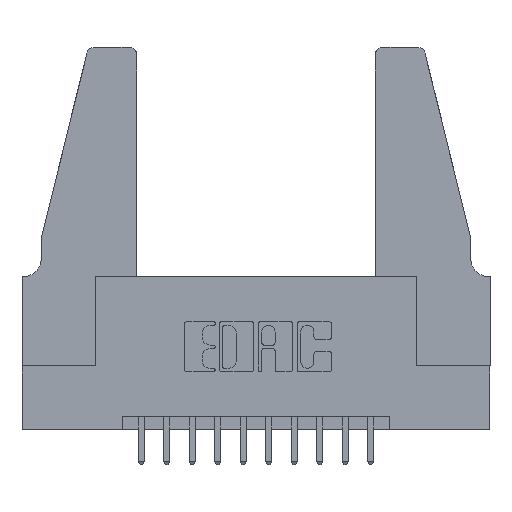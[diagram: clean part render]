
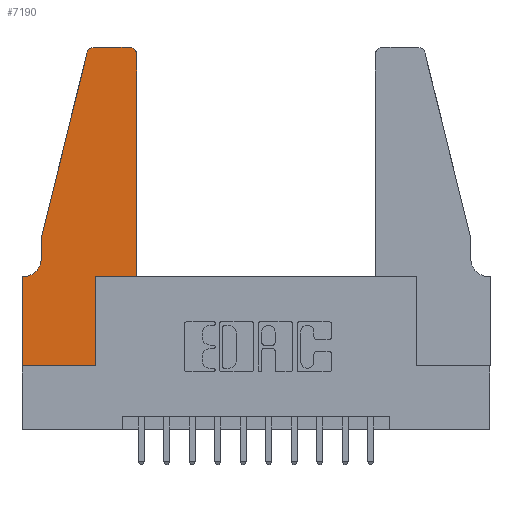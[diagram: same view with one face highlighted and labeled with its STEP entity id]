
A CAD part, top view. The second image highlights one B-rep face of the part: STEP entity #7190.
In plain terms, the highlighted planar face has unit normal (0, 0, 1).
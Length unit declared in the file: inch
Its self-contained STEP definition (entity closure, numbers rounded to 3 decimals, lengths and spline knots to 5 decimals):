
#106 = DIRECTION ( 'NONE',  ( 0., 0., 1. ) ) ;
#136 = CIRCLE ( 'NONE', #2397, 0.03 ) ;
#279 = DIRECTION ( 'NONE',  ( 1., 0., 0. ) ) ;
#528 = CARTESIAN_POINT ( 'NONE',  ( 0.4205, 1.22, 0.37 ) ) ;
#578 = ORIENTED_EDGE ( 'NONE', *, *, #6038, .T. ) ;
#714 = EDGE_CURVE ( 'NONE', #11721, #8937, #3862, .T. ) ;
#1007 = VERTEX_POINT ( 'NONE', #6798 ) ;
#1129 = ORIENTED_EDGE ( 'NONE', *, *, #714, .T. ) ;
#1143 = CARTESIAN_POINT ( 'NONE',  ( 0.2605, 1.25, 0.37 ) ) ;
#1186 = CIRCLE ( 'NONE', #14248, 0.03 ) ;
#1503 = LINE ( 'NONE', #11386, #5485 ) ;
#1522 = DIRECTION ( 'NONE',  ( 0., 0., 1. ) ) ;
#1539 = CARTESIAN_POINT ( 'NONE',  ( 0.0755, 0.42, 0.37 ) ) ;
#1570 = VECTOR ( 'NONE', #9834, 39.37008 ) ;
#1908 = VECTOR ( 'NONE', #6841, 39.37008 ) ;
#2187 = DIRECTION ( 'NONE',  ( 1., 0., 0. ) ) ;
#2288 = CARTESIAN_POINT ( 'NONE',  ( 0.0755, 0.5, 0.37 ) ) ;
#2299 = CARTESIAN_POINT ( 'NONE',  ( 0.25487, 1.22718, 0.37 ) ) ;
#2397 = AXIS2_PLACEMENT_3D ( 'NONE', #528, #12698, #13999 ) ;
#2449 = LINE ( 'NONE', #9709, #11997 ) ;
#2630 = CARTESIAN_POINT ( 'NONE',  ( 0., 0., 0.37 ) ) ;
#2727 = ORIENTED_EDGE ( 'NONE', *, *, #8529, .T. ) ;
#2796 = CARTESIAN_POINT ( 'NONE',  ( 0.284, 1.25, 0.37 ) ) ;
#3583 = VERTEX_POINT ( 'NONE', #2299 ) ;
#3639 = EDGE_CURVE ( 'NONE', #10085, #7294, #9770, .T. ) ;
#3790 = CARTESIAN_POINT ( 'NONE',  ( 0.284, 1.22, 0.37 ) ) ;
#3795 = ORIENTED_EDGE ( 'NONE', *, *, #13340, .T. ) ;
#3862 = LINE ( 'NONE', #8742, #6840 ) ;
#3880 = VECTOR ( 'NONE', #8883, 39.37008 ) ;
#3984 = CARTESIAN_POINT ( 'NONE',  ( 0., 0.35, 0.37 ) ) ;
#4193 = DIRECTION ( 'NONE',  ( 0., 0., -1. ) ) ;
#4283 = VERTEX_POINT ( 'NONE', #7846 ) ;
#4570 = DIRECTION ( 'NONE',  ( 0., 1., 0. ) ) ;
#4996 = LINE ( 'NONE', #10945, #10526 ) ;
#5485 = VECTOR ( 'NONE', #5853, 39.37008 ) ;
#5659 = EDGE_CURVE ( 'NONE', #4283, #10770, #13568, .T. ) ;
#5853 = DIRECTION ( 'NONE',  ( 1., 0., 0. ) ) ;
#6017 = VERTEX_POINT ( 'NONE', #10957 ) ;
#6038 = EDGE_CURVE ( 'NONE', #6017, #4283, #2449, .T. ) ;
#6058 = CARTESIAN_POINT ( 'NONE',  ( 0.0755, 0.35, 0.37 ) ) ;
#6085 = LINE ( 'NONE', #2288, #1570 ) ;
#6108 = DIRECTION ( 'NONE',  ( -1., 0., 0. ) ) ;
#6505 = ORIENTED_EDGE ( 'NONE', *, *, #8764, .T. ) ;
#6798 = CARTESIAN_POINT ( 'NONE',  ( 0.2865, 0., 0.37 ) ) ;
#6840 = VECTOR ( 'NONE', #9835, 39.37008 ) ;
#6841 = DIRECTION ( 'NONE',  ( -0.239, -0.971, 0. ) ) ;
#6954 = ORIENTED_EDGE ( 'NONE', *, *, #13692, .T. ) ;
#6960 = DIRECTION ( 'NONE',  ( 0., 1., 0. ) ) ;
#7078 = CARTESIAN_POINT ( 'NONE',  ( 0.4505, 1.22, 0.37 ) ) ;
#7080 = CIRCLE ( 'NONE', #7215, 0.07 ) ;
#7100 = CARTESIAN_POINT ( 'NONE',  ( 0.4205, 1.25, 0.37 ) ) ;
#7190 = ADVANCED_FACE ( 'NONE', ( #9505 ), #8804, .T. ) ;
#7215 = AXIS2_PLACEMENT_3D ( 'NONE', #9684, #4193, #13051 ) ;
#7294 = VERTEX_POINT ( 'NONE', #2796 ) ;
#7559 = DIRECTION ( 'NONE',  ( 1., 0., 0. ) ) ;
#7713 = ORIENTED_EDGE ( 'NONE', *, *, #13967, .T. ) ;
#7791 = EDGE_CURVE ( 'NONE', #7294, #3583, #1186, .T. ) ;
#7813 = LINE ( 'NONE', #8763, #1908 ) ;
#7846 = CARTESIAN_POINT ( 'NONE',  ( 0.4505, 0.35, 0.37 ) ) ;
#8526 = VERTEX_POINT ( 'NONE', #13048 ) ;
#8529 = EDGE_CURVE ( 'NONE', #1007, #6017, #4996, .T. ) ;
#8742 = CARTESIAN_POINT ( 'NONE',  ( 0., 0., 0.37 ) ) ;
#8763 = CARTESIAN_POINT ( 'NONE',  ( 0.0755, 0.5, 0.37 ) ) ;
#8764 = EDGE_CURVE ( 'NONE', #14022, #9669, #7080, .T. ) ;
#8804 = PLANE ( 'NONE',  #11836 ) ;
#8883 = DIRECTION ( 'NONE',  ( -1., 0., 0. ) ) ;
#8937 = VERTEX_POINT ( 'NONE', #2630 ) ;
#9067 = CARTESIAN_POINT ( 'NONE',  ( 0.0055, 0.35, 0.37 ) ) ;
#9285 = ORIENTED_EDGE ( 'NONE', *, *, #5659, .T. ) ;
#9505 = FACE_OUTER_BOUND ( 'NONE', #9744, .T. ) ;
#9669 = VERTEX_POINT ( 'NONE', #9067 ) ;
#9684 = CARTESIAN_POINT ( 'NONE',  ( 0.0055, 0.42, 0.37 ) ) ;
#9709 = CARTESIAN_POINT ( 'NONE',  ( 0.4505, 0.35, 0.37 ) ) ;
#9744 = EDGE_LOOP ( 'NONE', ( #12637, #13203, #13860, #10943, #6505, #7713, #1129, #6954, #2727, #578, #9285, #3795 ) ) ;
#9770 = LINE ( 'NONE', #1143, #3880 ) ;
#9795 = VECTOR ( 'NONE', #6108, 39.37008 ) ;
#9834 = DIRECTION ( 'NONE',  ( 0., -1., 0. ) ) ;
#9835 = DIRECTION ( 'NONE',  ( 0., -1., 0. ) ) ;
#10085 = VERTEX_POINT ( 'NONE', #7100 ) ;
#10526 = VECTOR ( 'NONE', #6960, 39.37008 ) ;
#10613 = VECTOR ( 'NONE', #4570, 39.37008 ) ;
#10770 = VERTEX_POINT ( 'NONE', #7078 ) ;
#10801 = EDGE_CURVE ( 'NONE', #8526, #14022, #6085, .T. ) ;
#10943 = ORIENTED_EDGE ( 'NONE', *, *, #10801, .T. ) ;
#10945 = CARTESIAN_POINT ( 'NONE',  ( 0.2865, 0.35, 0.37 ) ) ;
#10957 = CARTESIAN_POINT ( 'NONE',  ( 0.2865, 0.35, 0.37 ) ) ;
#11000 = EDGE_CURVE ( 'NONE', #3583, #8526, #7813, .T. ) ;
#11094 = CARTESIAN_POINT ( 'NONE',  ( 0., 0.35, 0.37 ) ) ;
#11386 = CARTESIAN_POINT ( 'NONE',  ( 0., 0., 0.37 ) ) ;
#11390 = LINE ( 'NONE', #6058, #9795 ) ;
#11721 = VERTEX_POINT ( 'NONE', #3984 ) ;
#11836 = AXIS2_PLACEMENT_3D ( 'NONE', #11094, #106, #2187 ) ;
#11997 = VECTOR ( 'NONE', #7559, 39.37008 ) ;
#12360 = CARTESIAN_POINT ( 'NONE',  ( 0.4505, 0.35, 0.37 ) ) ;
#12637 = ORIENTED_EDGE ( 'NONE', *, *, #3639, .T. ) ;
#12698 = DIRECTION ( 'NONE',  ( 0., 0., 1. ) ) ;
#13048 = CARTESIAN_POINT ( 'NONE',  ( 0.0755, 0.5, 0.37 ) ) ;
#13051 = DIRECTION ( 'NONE',  ( -1., 0., 0. ) ) ;
#13203 = ORIENTED_EDGE ( 'NONE', *, *, #7791, .T. ) ;
#13340 = EDGE_CURVE ( 'NONE', #10770, #10085, #136, .T. ) ;
#13568 = LINE ( 'NONE', #12360, #10613 ) ;
#13692 = EDGE_CURVE ( 'NONE', #8937, #1007, #1503, .T. ) ;
#13860 = ORIENTED_EDGE ( 'NONE', *, *, #11000, .T. ) ;
#13967 = EDGE_CURVE ( 'NONE', #9669, #11721, #11390, .T. ) ;
#13999 = DIRECTION ( 'NONE',  ( 1., 0., 0. ) ) ;
#14022 = VERTEX_POINT ( 'NONE', #1539 ) ;
#14248 = AXIS2_PLACEMENT_3D ( 'NONE', #3790, #1522, #279 ) ;
